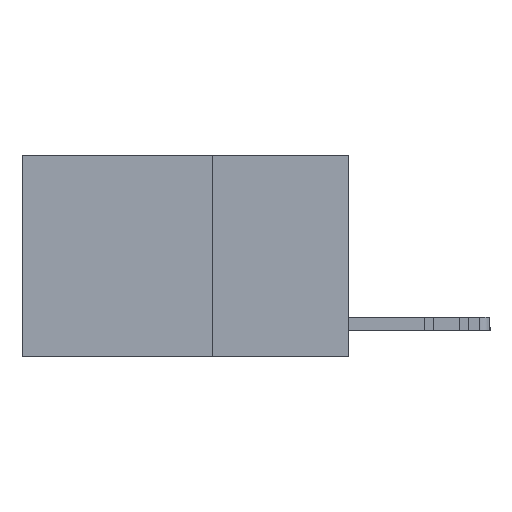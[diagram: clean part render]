
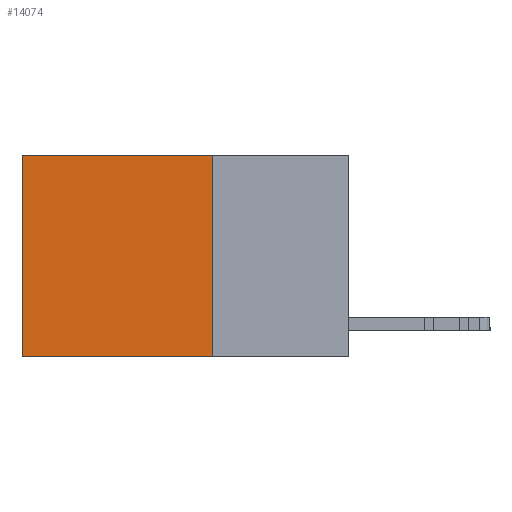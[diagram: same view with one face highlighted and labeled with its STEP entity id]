
A CAD part, left-side view. The second image highlights one B-rep face of the part: STEP entity #14074.
In plain terms, the highlighted planar face has unit normal (-1, 0, 0).
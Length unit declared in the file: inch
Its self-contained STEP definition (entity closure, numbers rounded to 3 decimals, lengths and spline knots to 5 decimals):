
#397 = VERTEX_POINT ( 'NONE', #10266 ) ;
#1568 = ORIENTED_EDGE ( 'NONE', *, *, #20241, .T. ) ;
#2752 = EDGE_LOOP ( 'NONE', ( #17979, #21602, #22156, #1568 ) ) ;
#3587 = VERTEX_POINT ( 'NONE', #17284 ) ;
#4455 = VERTEX_POINT ( 'NONE', #8548 ) ;
#4526 = CARTESIAN_POINT ( 'NONE',  ( 0.2625, 0.25, 0. ) ) ;
#7925 = CARTESIAN_POINT ( 'NONE',  ( 0.2625, 0.6, 0. ) ) ;
#8548 = CARTESIAN_POINT ( 'NONE',  ( 0.2625, 0.25, 0. ) ) ;
#9392 = LINE ( 'NONE', #18070, #15529 ) ;
#10175 = CARTESIAN_POINT ( 'NONE',  ( 0.2625, 0.25, 0. ) ) ;
#10266 = CARTESIAN_POINT ( 'NONE',  ( 0.2625, 0.6, 0. ) ) ;
#10801 = VECTOR ( 'NONE', #21435, 39.37008 ) ;
#12301 = LINE ( 'NONE', #10175, #19455 ) ;
#12893 = VECTOR ( 'NONE', #16007, 39.37008 ) ;
#13647 = EDGE_CURVE ( 'NONE', #18916, #3587, #9392, .T. ) ;
#14074 = ADVANCED_FACE ( 'NONE', ( #26584 ), #16034, .F. ) ;
#14606 = LINE ( 'NONE', #7925, #10801 ) ;
#15529 = VECTOR ( 'NONE', #22611, 39.37008 ) ;
#15870 = CARTESIAN_POINT ( 'NONE',  ( 0.2625, 0.25, 0. ) ) ;
#15903 = DIRECTION ( 'NONE',  ( 1., 0., 0. ) ) ;
#16007 = DIRECTION ( 'NONE',  ( 0., 1., 0. ) ) ;
#16034 = PLANE ( 'NONE',  #25552 ) ;
#17015 = CARTESIAN_POINT ( 'NONE',  ( 0.2625, 0.25, -0.37 ) ) ;
#17284 = CARTESIAN_POINT ( 'NONE',  ( 0.2625, 0.6, -0.37 ) ) ;
#17979 = ORIENTED_EDGE ( 'NONE', *, *, #26862, .T. ) ;
#18070 = CARTESIAN_POINT ( 'NONE',  ( 0.2625, 0.25, -0.37 ) ) ;
#18916 = VERTEX_POINT ( 'NONE', #17015 ) ;
#19455 = VECTOR ( 'NONE', #20983, 39.37008 ) ;
#20241 = EDGE_CURVE ( 'NONE', #4455, #397, #24422, .T. ) ;
#20983 = DIRECTION ( 'NONE',  ( 0., 0., -1. ) ) ;
#21435 = DIRECTION ( 'NONE',  ( 0., 0., -1. ) ) ;
#21602 = ORIENTED_EDGE ( 'NONE', *, *, #13647, .F. ) ;
#22156 = ORIENTED_EDGE ( 'NONE', *, *, #25358, .F. ) ;
#22611 = DIRECTION ( 'NONE',  ( 0., 1., 0. ) ) ;
#24422 = LINE ( 'NONE', #15870, #12893 ) ;
#24601 = DIRECTION ( 'NONE',  ( 0., 0., -1. ) ) ;
#25358 = EDGE_CURVE ( 'NONE', #4455, #18916, #12301, .T. ) ;
#25552 = AXIS2_PLACEMENT_3D ( 'NONE', #4526, #15903, #24601 ) ;
#26584 = FACE_OUTER_BOUND ( 'NONE', #2752, .T. ) ;
#26862 = EDGE_CURVE ( 'NONE', #397, #3587, #14606, .T. ) ;
